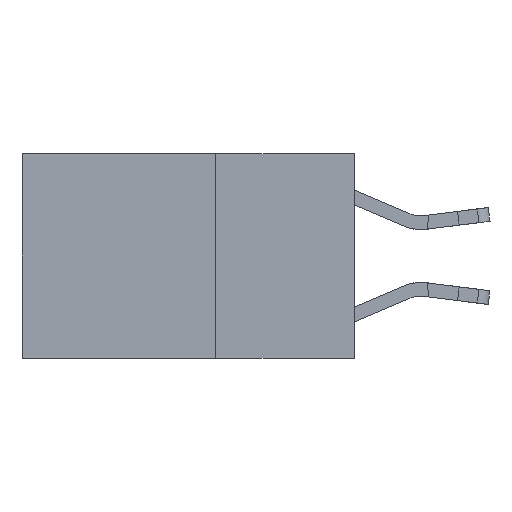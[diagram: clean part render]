
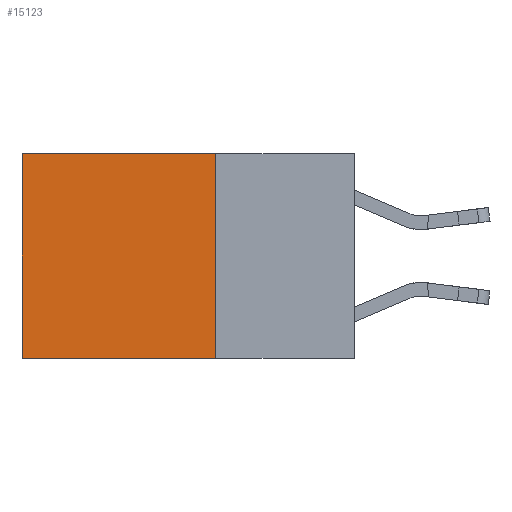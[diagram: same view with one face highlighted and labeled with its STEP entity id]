
A CAD part, left-side view. The second image highlights one B-rep face of the part: STEP entity #15123.
In plain terms, the highlighted planar face has unit normal (-1, 0, 0).
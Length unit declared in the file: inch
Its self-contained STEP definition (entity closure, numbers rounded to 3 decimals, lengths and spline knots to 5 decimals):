
#537 = VECTOR ( 'NONE', #11041, 39.37008 ) ;
#826 = LINE ( 'NONE', #15925, #15598 ) ;
#1127 = VERTEX_POINT ( 'NONE', #12733 ) ;
#1149 = DIRECTION ( 'NONE',  ( 0., 0., -1. ) ) ;
#1459 = LINE ( 'NONE', #13862, #537 ) ;
#1652 = EDGE_CURVE ( 'NONE', #14435, #1127, #826, .T. ) ;
#3893 = LINE ( 'NONE', #17222, #14837 ) ;
#4582 = CARTESIAN_POINT ( 'NONE',  ( 0.2625, 0.25, 0. ) ) ;
#4711 = EDGE_CURVE ( 'NONE', #6882, #5859, #5916, .T. ) ;
#5484 = CARTESIAN_POINT ( 'NONE',  ( 0.2625, 0.6, 0. ) ) ;
#5859 = VERTEX_POINT ( 'NONE', #5484 ) ;
#5916 = LINE ( 'NONE', #4582, #16777 ) ;
#6093 = AXIS2_PLACEMENT_3D ( 'NONE', #18181, #9815, #1149 ) ;
#6882 = VERTEX_POINT ( 'NONE', #13666 ) ;
#7356 = DIRECTION ( 'NONE',  ( 0., 0., -1. ) ) ;
#8357 = PLANE ( 'NONE',  #6093 ) ;
#9194 = EDGE_CURVE ( 'NONE', #6882, #14435, #1459, .T. ) ;
#9414 = CARTESIAN_POINT ( 'NONE',  ( 0.2625, 0.25, -0.37 ) ) ;
#9815 = DIRECTION ( 'NONE',  ( 1., 0., 0. ) ) ;
#10092 = ORIENTED_EDGE ( 'NONE', *, *, #1652, .F. ) ;
#11041 = DIRECTION ( 'NONE',  ( 0., 0., -1. ) ) ;
#11423 = ORIENTED_EDGE ( 'NONE', *, *, #15344, .T. ) ;
#11728 = ORIENTED_EDGE ( 'NONE', *, *, #4711, .T. ) ;
#11744 = FACE_OUTER_BOUND ( 'NONE', #16575, .T. ) ;
#12733 = CARTESIAN_POINT ( 'NONE',  ( 0.2625, 0.6, -0.37 ) ) ;
#13122 = DIRECTION ( 'NONE',  ( 0., 1., 0. ) ) ;
#13666 = CARTESIAN_POINT ( 'NONE',  ( 0.2625, 0.25, 0. ) ) ;
#13862 = CARTESIAN_POINT ( 'NONE',  ( 0.2625, 0.25, 0. ) ) ;
#14435 = VERTEX_POINT ( 'NONE', #9414 ) ;
#14837 = VECTOR ( 'NONE', #7356, 39.37008 ) ;
#15123 = ADVANCED_FACE ( 'NONE', ( #11744 ), #8357, .F. ) ;
#15344 = EDGE_CURVE ( 'NONE', #5859, #1127, #3893, .T. ) ;
#15598 = VECTOR ( 'NONE', #17320, 39.37008 ) ;
#15925 = CARTESIAN_POINT ( 'NONE',  ( 0.2625, 0.25, -0.37 ) ) ;
#16575 = EDGE_LOOP ( 'NONE', ( #11423, #10092, #17954, #11728 ) ) ;
#16777 = VECTOR ( 'NONE', #13122, 39.37008 ) ;
#17222 = CARTESIAN_POINT ( 'NONE',  ( 0.2625, 0.6, 0. ) ) ;
#17320 = DIRECTION ( 'NONE',  ( 0., 1., 0. ) ) ;
#17954 = ORIENTED_EDGE ( 'NONE', *, *, #9194, .F. ) ;
#18181 = CARTESIAN_POINT ( 'NONE',  ( 0.2625, 0.25, 0. ) ) ;
